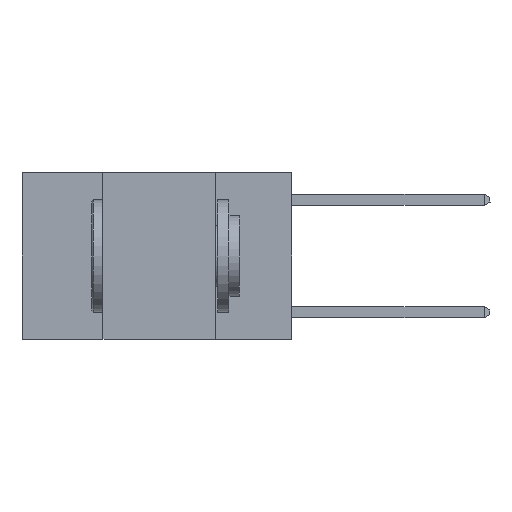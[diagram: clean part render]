
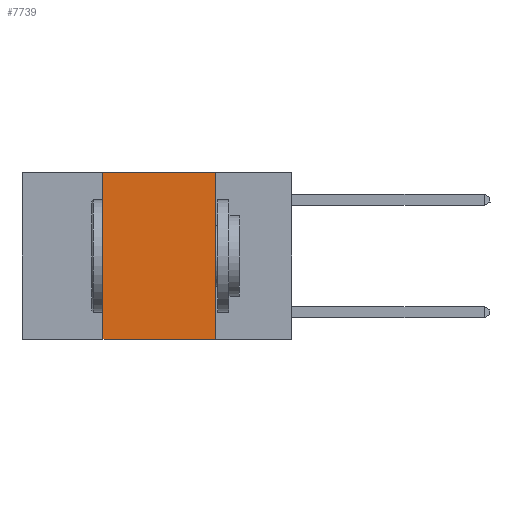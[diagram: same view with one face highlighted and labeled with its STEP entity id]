
A CAD part, left-side view. The second image highlights one B-rep face of the part: STEP entity #7739.
In plain terms, the highlighted planar face has unit normal (-1, 0, 0).
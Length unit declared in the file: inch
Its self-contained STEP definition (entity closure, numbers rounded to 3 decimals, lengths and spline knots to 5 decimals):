
#411 = VERTEX_POINT ( 'NONE', #15933 ) ;
#745 = DIRECTION ( 'NONE',  ( 0., 0., 1. ) ) ;
#1684 = ORIENTED_EDGE ( 'NONE', *, *, #21035, .F. ) ;
#2262 = ORIENTED_EDGE ( 'NONE', *, *, #22357, .F. ) ;
#2457 = ORIENTED_EDGE ( 'NONE', *, *, #22209, .F. ) ;
#2865 = ORIENTED_EDGE ( 'NONE', *, *, #23426, .T. ) ;
#2989 = FACE_OUTER_BOUND ( 'NONE', #23520, .T. ) ;
#4212 = CARTESIAN_POINT ( 'NONE',  ( 0., 0.17, -0.37 ) ) ;
#4888 = LINE ( 'NONE', #16062, #23929 ) ;
#5033 = DIRECTION ( 'NONE',  ( 0., 0., -1. ) ) ;
#5752 = LINE ( 'NONE', #6866, #15041 ) ;
#6866 = CARTESIAN_POINT ( 'NONE',  ( 0., 0.6, 0. ) ) ;
#6918 = CARTESIAN_POINT ( 'NONE',  ( 0., 0.17, 0. ) ) ;
#7739 = ADVANCED_FACE ( 'NONE', ( #2989 ), #19091, .F. ) ;
#8725 = DIRECTION ( 'NONE',  ( 0., -1., 0. ) ) ;
#8748 = VERTEX_POINT ( 'NONE', #4212 ) ;
#9853 = DIRECTION ( 'NONE',  ( 0., 0., -1. ) ) ;
#10219 = VECTOR ( 'NONE', #5033, 39.37008 ) ;
#13653 = CARTESIAN_POINT ( 'NONE',  ( 0., 0.42, -0.37 ) ) ;
#13837 = CARTESIAN_POINT ( 'NONE',  ( 0., 0.42, 0. ) ) ;
#14432 = AXIS2_PLACEMENT_3D ( 'NONE', #17199, #20935, #9853 ) ;
#15041 = VECTOR ( 'NONE', #8725, 39.37008 ) ;
#15680 = LINE ( 'NONE', #6918, #10219 ) ;
#15933 = CARTESIAN_POINT ( 'NONE',  ( 0., 0.17, 0. ) ) ;
#16062 = CARTESIAN_POINT ( 'NONE',  ( 0., 0.6, -0.37 ) ) ;
#17199 = CARTESIAN_POINT ( 'NONE',  ( 0., 0.6, 0. ) ) ;
#17945 = VECTOR ( 'NONE', #745, 39.37008 ) ;
#17996 = CARTESIAN_POINT ( 'NONE',  ( 0., 0.42, 0. ) ) ;
#19091 = PLANE ( 'NONE',  #14432 ) ;
#20081 = VERTEX_POINT ( 'NONE', #13653 ) ;
#20935 = DIRECTION ( 'NONE',  ( 1., 0., 0. ) ) ;
#21035 = EDGE_CURVE ( 'NONE', #411, #8748, #15680, .T. ) ;
#22209 = EDGE_CURVE ( 'NONE', #20081, #23465, #22797, .T. ) ;
#22357 = EDGE_CURVE ( 'NONE', #23465, #411, #5752, .T. ) ;
#22797 = LINE ( 'NONE', #13837, #17945 ) ;
#23419 = DIRECTION ( 'NONE',  ( 0., -1., 0. ) ) ;
#23426 = EDGE_CURVE ( 'NONE', #20081, #8748, #4888, .T. ) ;
#23465 = VERTEX_POINT ( 'NONE', #17996 ) ;
#23520 = EDGE_LOOP ( 'NONE', ( #1684, #2262, #2457, #2865 ) ) ;
#23929 = VECTOR ( 'NONE', #23419, 39.37008 ) ;
